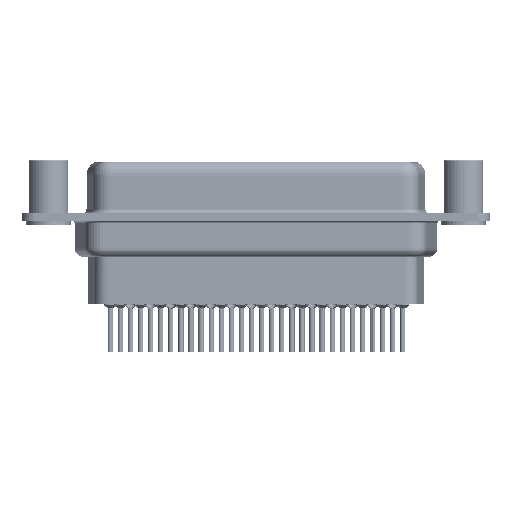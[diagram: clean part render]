
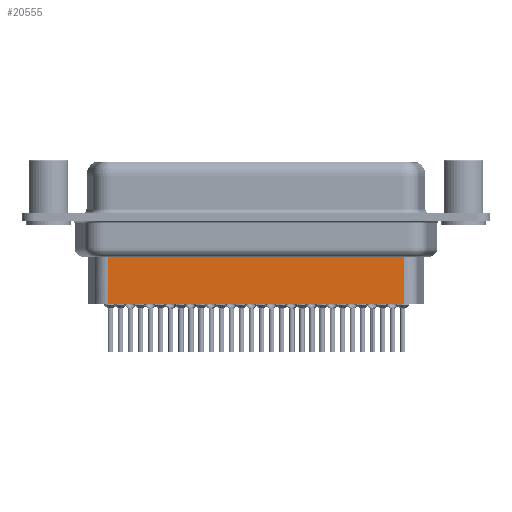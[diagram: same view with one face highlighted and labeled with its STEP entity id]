
A CAD part, front view. The second image highlights one B-rep face of the part: STEP entity #20555.
In plain terms, the highlighted planar face has unit normal (0, -1, 0).
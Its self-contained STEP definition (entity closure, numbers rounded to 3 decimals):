
#745 = VECTOR ( 'NONE', #29115, 1000. ) ;
#1617 = DIRECTION ( 'NONE',  ( -1., 0., 0. ) ) ;
#1785 = DIRECTION ( 'NONE',  ( 1., 0., 0. ) ) ;
#2747 = CARTESIAN_POINT ( 'NONE',  ( 40.339, -3.5, -3.1 ) ) ;
#3961 = ORIENTED_EDGE ( 'NONE', *, *, #9255, .F. ) ;
#4110 = VECTOR ( 'NONE', #20310, 1000. ) ;
#4269 = CARTESIAN_POINT ( 'NONE',  ( 6.701, -3.5, -9.85 ) ) ;
#4388 = ORIENTED_EDGE ( 'NONE', *, *, #37548, .T. ) ;
#5007 = CARTESIAN_POINT ( 'NONE',  ( 6.701, -3.5, -4.097 ) ) ;
#5277 = VERTEX_POINT ( 'NONE', #5007 ) ;
#6132 = VERTEX_POINT ( 'NONE', #15271 ) ;
#6771 = VECTOR ( 'NONE', #21252, 1000. ) ;
#9255 = EDGE_CURVE ( 'NONE', #6132, #24647, #13922, .T. ) ;
#10634 = AXIS2_PLACEMENT_3D ( 'NONE', #14528, #14124, #1785 ) ;
#12622 = VECTOR ( 'NONE', #1617, 1000. ) ;
#13922 = LINE ( 'NONE', #4269, #745 ) ;
#14124 = DIRECTION ( 'NONE',  ( 0., -1., 0. ) ) ;
#14528 = CARTESIAN_POINT ( 'NONE',  ( 6.701, -3.5, -3.1 ) ) ;
#15271 = CARTESIAN_POINT ( 'NONE',  ( 40.339, -3.5, -9.85 ) ) ;
#17429 = CARTESIAN_POINT ( 'NONE',  ( 6.454, -3.5, -4.097 ) ) ;
#17844 = LINE ( 'NONE', #23372, #4110 ) ;
#18412 = EDGE_LOOP ( 'NONE', ( #33933, #4388, #37244, #3961 ) ) ;
#18931 = CARTESIAN_POINT ( 'NONE',  ( 40.339, -3.5, -4.097 ) ) ;
#20310 = DIRECTION ( 'NONE',  ( 0., 0., -1. ) ) ;
#20555 = ADVANCED_FACE ( 'NONE', ( #26437 ), #38998, .T. ) ;
#21252 = DIRECTION ( 'NONE',  ( 0., 0., -1. ) ) ;
#22293 = EDGE_CURVE ( 'NONE', #22698, #6132, #33964, .T. ) ;
#22698 = VERTEX_POINT ( 'NONE', #18931 ) ;
#23372 = CARTESIAN_POINT ( 'NONE',  ( 6.701, -3.5, -3.1 ) ) ;
#24647 = VERTEX_POINT ( 'NONE', #32998 ) ;
#26437 = FACE_OUTER_BOUND ( 'NONE', #18412, .T. ) ;
#26458 = LINE ( 'NONE', #17429, #12622 ) ;
#29115 = DIRECTION ( 'NONE',  ( -1., 0., 0. ) ) ;
#32998 = CARTESIAN_POINT ( 'NONE',  ( 6.701, -3.5, -9.85 ) ) ;
#33933 = ORIENTED_EDGE ( 'NONE', *, *, #22293, .F. ) ;
#33964 = LINE ( 'NONE', #2747, #6771 ) ;
#37244 = ORIENTED_EDGE ( 'NONE', *, *, #37500, .T. ) ;
#37500 = EDGE_CURVE ( 'NONE', #5277, #24647, #17844, .T. ) ;
#37548 = EDGE_CURVE ( 'NONE', #22698, #5277, #26458, .T. ) ;
#38998 = PLANE ( 'NONE',  #10634 ) ;
